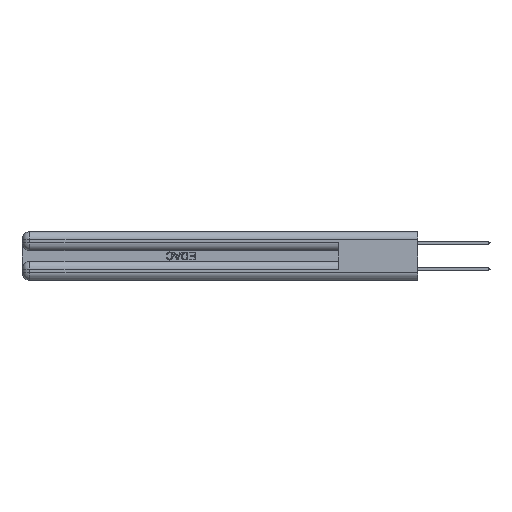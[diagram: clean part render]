
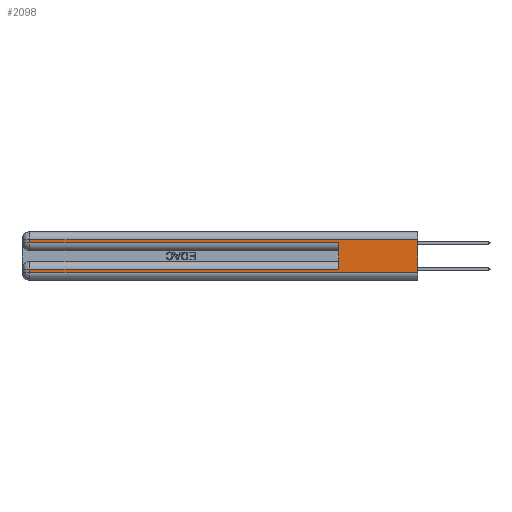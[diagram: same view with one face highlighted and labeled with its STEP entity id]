
A CAD part, left-side view. The second image highlights one B-rep face of the part: STEP entity #2098.
In plain terms, the highlighted planar face has unit normal (-1, 0, 0).
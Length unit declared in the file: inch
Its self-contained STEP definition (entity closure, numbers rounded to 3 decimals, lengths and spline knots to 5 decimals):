
#10 = DIRECTION ( 'NONE',  ( 0., -1., 0. ) ) ;
#2098 = ADVANCED_FACE ( 'NONE', ( #40261 ), #35003, .F. ) ;
#3474 = EDGE_CURVE ( 'NONE', #12933, #23440, #29439, .T. ) ;
#4673 = VERTEX_POINT ( 'NONE', #26066 ) ;
#5814 = ORIENTED_EDGE ( 'NONE', *, *, #34020, .T. ) ;
#5873 = VECTOR ( 'NONE', #50618, 39.37008 ) ;
#6094 = CARTESIAN_POINT ( 'NONE',  ( 0., 0., 0.31 ) ) ;
#6739 = ORIENTED_EDGE ( 'NONE', *, *, #30177, .T. ) ;
#8825 = VERTEX_POINT ( 'NONE', #29321 ) ;
#10211 = VERTEX_POINT ( 'NONE', #12315 ) ;
#10433 = CARTESIAN_POINT ( 'NONE',  ( 0., 0., 0.06 ) ) ;
#11559 = LINE ( 'NONE', #20839, #30619 ) ;
#12059 = DIRECTION ( 'NONE',  ( 0., 0., 1. ) ) ;
#12167 = VECTOR ( 'NONE', #10, 39.37008 ) ;
#12313 = EDGE_CURVE ( 'NONE', #46006, #32228, #51981, .T. ) ;
#12315 = CARTESIAN_POINT ( 'NONE',  ( 0., 2.94, 0.31 ) ) ;
#12763 = DIRECTION ( 'NONE',  ( 0., 1., 0. ) ) ;
#12829 = VECTOR ( 'NONE', #27730, 39.37008 ) ;
#12933 = VERTEX_POINT ( 'NONE', #14300 ) ;
#13251 = VECTOR ( 'NONE', #50211, 39.37008 ) ;
#14300 = CARTESIAN_POINT ( 'NONE',  ( 0., 0.6, 0.085 ) ) ;
#14891 = DIRECTION ( 'NONE',  ( 0., 0., -1. ) ) ;
#17308 = CARTESIAN_POINT ( 'NONE',  ( 0., 2.94, 0.085 ) ) ;
#17625 = ORIENTED_EDGE ( 'NONE', *, *, #3474, .F. ) ;
#18709 = VECTOR ( 'NONE', #12059, 39.37008 ) ;
#19511 = CARTESIAN_POINT ( 'NONE',  ( 0., 2.94, 0.37 ) ) ;
#19652 = ORIENTED_EDGE ( 'NONE', *, *, #32801, .T. ) ;
#19889 = EDGE_CURVE ( 'NONE', #12933, #42551, #11559, .T. ) ;
#20839 = CARTESIAN_POINT ( 'NONE',  ( 0., 0., 0.085 ) ) ;
#21679 = ORIENTED_EDGE ( 'NONE', *, *, #19889, .T. ) ;
#22302 = CARTESIAN_POINT ( 'NONE',  ( 0., 0., 0.37 ) ) ;
#23440 = VERTEX_POINT ( 'NONE', #35039 ) ;
#23675 = CARTESIAN_POINT ( 'NONE',  ( 0., 2.94, 0.37 ) ) ;
#24440 = ORIENTED_EDGE ( 'NONE', *, *, #12313, .F. ) ;
#24719 = CARTESIAN_POINT ( 'NONE',  ( 0., 0., 0.285 ) ) ;
#26066 = CARTESIAN_POINT ( 'NONE',  ( 0., 2.94, 0.06 ) ) ;
#26178 = CARTESIAN_POINT ( 'NONE',  ( 0., 0., 0.06 ) ) ;
#26744 = LINE ( 'NONE', #19511, #48065 ) ;
#27730 = DIRECTION ( 'NONE',  ( 0., 0., -1. ) ) ;
#29321 = CARTESIAN_POINT ( 'NONE',  ( 0., 2.94, 0.285 ) ) ;
#29439 = LINE ( 'NONE', #36299, #18709 ) ;
#30177 = EDGE_CURVE ( 'NONE', #4673, #32228, #45427, .T. ) ;
#30619 = VECTOR ( 'NONE', #12763, 39.37008 ) ;
#31916 = VECTOR ( 'NONE', #46330, 39.37008 ) ;
#32228 = VERTEX_POINT ( 'NONE', #10433 ) ;
#32801 = EDGE_CURVE ( 'NONE', #46006, #10211, #51405, .T. ) ;
#33721 = LINE ( 'NONE', #24719, #12167 ) ;
#34020 = EDGE_CURVE ( 'NONE', #8825, #23440, #33721, .T. ) ;
#35003 = PLANE ( 'NONE',  #49063 ) ;
#35039 = CARTESIAN_POINT ( 'NONE',  ( 0., 0.6, 0.285 ) ) ;
#36299 = CARTESIAN_POINT ( 'NONE',  ( 0., 0.6, 0.145 ) ) ;
#37773 = CARTESIAN_POINT ( 'NONE',  ( 0., 0., 0.31 ) ) ;
#39055 = DIRECTION ( 'NONE',  ( 1., 0., 0. ) ) ;
#39350 = ORIENTED_EDGE ( 'NONE', *, *, #50271, .T. ) ;
#39633 = EDGE_CURVE ( 'NONE', #10211, #8825, #26744, .T. ) ;
#39706 = ORIENTED_EDGE ( 'NONE', *, *, #39633, .T. ) ;
#39804 = EDGE_LOOP ( 'NONE', ( #24440, #19652, #39706, #5814, #17625, #21679, #39350, #6739 ) ) ;
#40261 = FACE_OUTER_BOUND ( 'NONE', #39804, .T. ) ;
#42551 = VERTEX_POINT ( 'NONE', #17308 ) ;
#45035 = LINE ( 'NONE', #23675, #12829 ) ;
#45427 = LINE ( 'NONE', #26178, #13251 ) ;
#46006 = VERTEX_POINT ( 'NONE', #37773 ) ;
#46330 = DIRECTION ( 'NONE',  ( 0., 0., -1. ) ) ;
#46906 = CARTESIAN_POINT ( 'NONE',  ( 0., 0., 0.37 ) ) ;
#47574 = DIRECTION ( 'NONE',  ( 0., 0., -1. ) ) ;
#48065 = VECTOR ( 'NONE', #47574, 39.37008 ) ;
#49063 = AXIS2_PLACEMENT_3D ( 'NONE', #46906, #39055, #14891 ) ;
#50211 = DIRECTION ( 'NONE',  ( 0., -1., 0. ) ) ;
#50271 = EDGE_CURVE ( 'NONE', #42551, #4673, #45035, .T. ) ;
#50618 = DIRECTION ( 'NONE',  ( 0., 1., 0. ) ) ;
#51405 = LINE ( 'NONE', #6094, #5873 ) ;
#51981 = LINE ( 'NONE', #22302, #31916 ) ;
